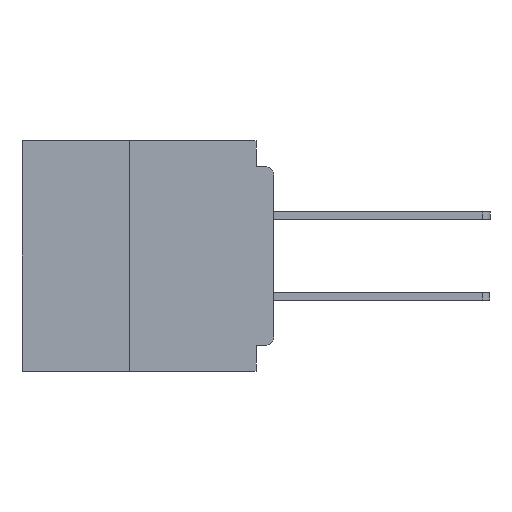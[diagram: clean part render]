
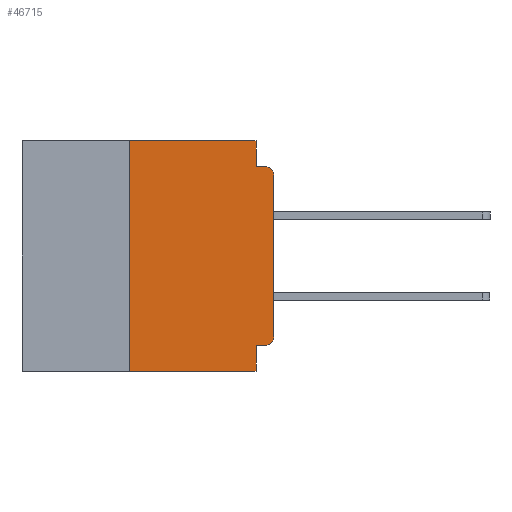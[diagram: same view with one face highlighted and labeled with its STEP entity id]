
A CAD part, left-side view. The second image highlights one B-rep face of the part: STEP entity #46715.
In plain terms, the highlighted planar face has unit normal (-1, 0, 0).
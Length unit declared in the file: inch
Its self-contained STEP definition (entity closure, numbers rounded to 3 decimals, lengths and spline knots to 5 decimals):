
#1260 = ORIENTED_EDGE ( 'NONE', *, *, #4065, .F. ) ;
#1386 = DIRECTION ( 'NONE',  ( 0., 0., -1. ) ) ;
#2509 = CARTESIAN_POINT ( 'NONE',  ( 0., 0.015, -0.355 ) ) ;
#2570 = VERTEX_POINT ( 'NONE', #18987 ) ;
#2714 = LINE ( 'NONE', #21252, #49783 ) ;
#4065 = EDGE_CURVE ( 'NONE', #26588, #33349, #13786, .T. ) ;
#6984 = LINE ( 'NONE', #49546, #52693 ) ;
#7723 = CARTESIAN_POINT ( 'NONE',  ( 0., 0.437, 0. ) ) ;
#8482 = ORIENTED_EDGE ( 'NONE', *, *, #28349, .F. ) ;
#8968 = ORIENTED_EDGE ( 'NONE', *, *, #21781, .T. ) ;
#9814 = LINE ( 'NONE', #50591, #43721 ) ;
#10561 = VERTEX_POINT ( 'NONE', #35014 ) ;
#11578 = VERTEX_POINT ( 'NONE', #30526 ) ;
#11749 = DIRECTION ( 'NONE',  ( 0., 1., 0. ) ) ;
#12349 = EDGE_CURVE ( 'NONE', #39639, #48345, #39547, .T. ) ;
#13540 = LINE ( 'NONE', #41100, #22592 ) ;
#13786 = LINE ( 'NONE', #43522, #46334 ) ;
#15173 = CARTESIAN_POINT ( 'NONE',  ( 0., 0.25, -0.4 ) ) ;
#15641 = DIRECTION ( 'NONE',  ( -1., 0., 0. ) ) ;
#17525 = CARTESIAN_POINT ( 'NONE',  ( 0., 0., -0.045 ) ) ;
#17658 = VERTEX_POINT ( 'NONE', #15173 ) ;
#18987 = CARTESIAN_POINT ( 'NONE',  ( 0., 0.015, -0.045 ) ) ;
#21252 = CARTESIAN_POINT ( 'NONE',  ( 0., 0.25, -0.4 ) ) ;
#21430 = ORIENTED_EDGE ( 'NONE', *, *, #26147, .F. ) ;
#21475 = CARTESIAN_POINT ( 'NONE',  ( 0., 0., 0. ) ) ;
#21781 = EDGE_CURVE ( 'NONE', #17658, #23267, #9814, .T. ) ;
#22251 = EDGE_CURVE ( 'NONE', #10561, #26588, #6984, .T. ) ;
#22592 = VECTOR ( 'NONE', #23510, 39.37008 ) ;
#23130 = EDGE_LOOP ( 'NONE', ( #33157, #50341, #8482, #1260, #29506, #32624, #8968, #35141, #21430, #47176 ) ) ;
#23249 = LINE ( 'NONE', #24923, #57124 ) ;
#23267 = VERTEX_POINT ( 'NONE', #32295 ) ;
#23510 = DIRECTION ( 'NONE',  ( 0., 0., -1. ) ) ;
#24923 = CARTESIAN_POINT ( 'NONE',  ( 0., 0., -0.355 ) ) ;
#25291 = DIRECTION ( 'NONE',  ( 0., 0., 1. ) ) ;
#25569 = PLANE ( 'NONE',  #44986 ) ;
#26147 = EDGE_CURVE ( 'NONE', #39639, #41150, #23249, .T. ) ;
#26588 = VERTEX_POINT ( 'NONE', #54233 ) ;
#27921 = DIRECTION ( 'NONE',  ( -1., 0., 0. ) ) ;
#28349 = EDGE_CURVE ( 'NONE', #33349, #2570, #48219, .T. ) ;
#28579 = EDGE_CURVE ( 'NONE', #41150, #23267, #13540, .T. ) ;
#28597 = CARTESIAN_POINT ( 'NONE',  ( 0., 0.031, -0.045 ) ) ;
#28895 = FACE_OUTER_BOUND ( 'NONE', #23130, .T. ) ;
#29026 = CARTESIAN_POINT ( 'NONE',  ( 0., 0.031, -0.355 ) ) ;
#29506 = ORIENTED_EDGE ( 'NONE', *, *, #22251, .F. ) ;
#30049 = DIRECTION ( 'NONE',  ( 0., 0., -1. ) ) ;
#30526 = CARTESIAN_POINT ( 'NONE',  ( 0., 0., -0.06 ) ) ;
#30920 = DIRECTION ( 'NONE',  ( 0., -1., 0. ) ) ;
#31997 = DIRECTION ( 'NONE',  ( 0., -1., 0. ) ) ;
#32295 = CARTESIAN_POINT ( 'NONE',  ( 0., 0.031, -0.4 ) ) ;
#32624 = ORIENTED_EDGE ( 'NONE', *, *, #51682, .F. ) ;
#33157 = ORIENTED_EDGE ( 'NONE', *, *, #35260, .T. ) ;
#33349 = VERTEX_POINT ( 'NONE', #28597 ) ;
#33749 = VECTOR ( 'NONE', #30920, 39.37008 ) ;
#35014 = CARTESIAN_POINT ( 'NONE',  ( 0., 0.25, 0. ) ) ;
#35064 = EDGE_CURVE ( 'NONE', #11578, #2570, #53491, .T. ) ;
#35141 = ORIENTED_EDGE ( 'NONE', *, *, #28579, .F. ) ;
#35260 = EDGE_CURVE ( 'NONE', #48345, #11578, #42392, .T. ) ;
#37229 = DIRECTION ( 'NONE',  ( 0., -1., 0. ) ) ;
#37273 = AXIS2_PLACEMENT_3D ( 'NONE', #42157, #15641, #46585 ) ;
#39547 = CIRCLE ( 'NONE', #56063, 0.015 ) ;
#39639 = VERTEX_POINT ( 'NONE', #2509 ) ;
#41034 = VECTOR ( 'NONE', #52397, 39.37008 ) ;
#41100 = CARTESIAN_POINT ( 'NONE',  ( 0., 0.031, -0.4 ) ) ;
#41150 = VERTEX_POINT ( 'NONE', #29026 ) ;
#42157 = CARTESIAN_POINT ( 'NONE',  ( 0., 0.015, -0.06 ) ) ;
#42392 = LINE ( 'NONE', #21475, #41034 ) ;
#43522 = CARTESIAN_POINT ( 'NONE',  ( 0., 0.031, 0. ) ) ;
#43708 = DIRECTION ( 'NONE',  ( 0., 0., -1. ) ) ;
#43721 = VECTOR ( 'NONE', #37229, 39.37008 ) ;
#44986 = AXIS2_PLACEMENT_3D ( 'NONE', #7723, #56482, #30049 ) ;
#46334 = VECTOR ( 'NONE', #43708, 39.37008 ) ;
#46585 = DIRECTION ( 'NONE',  ( 0., 0., -1. ) ) ;
#46715 = ADVANCED_FACE ( 'NONE', ( #28895 ), #25569, .F. ) ;
#47176 = ORIENTED_EDGE ( 'NONE', *, *, #12349, .T. ) ;
#48219 = LINE ( 'NONE', #17525, #33749 ) ;
#48345 = VERTEX_POINT ( 'NONE', #50555 ) ;
#49546 = CARTESIAN_POINT ( 'NONE',  ( 0., 0.437, 0. ) ) ;
#49783 = VECTOR ( 'NONE', #25291, 39.37008 ) ;
#50341 = ORIENTED_EDGE ( 'NONE', *, *, #35064, .T. ) ;
#50555 = CARTESIAN_POINT ( 'NONE',  ( 0., 0., -0.34 ) ) ;
#50591 = CARTESIAN_POINT ( 'NONE',  ( 0., 0.437, -0.4 ) ) ;
#51682 = EDGE_CURVE ( 'NONE', #17658, #10561, #2714, .T. ) ;
#52397 = DIRECTION ( 'NONE',  ( 0., 0., 1. ) ) ;
#52693 = VECTOR ( 'NONE', #31997, 39.37008 ) ;
#53491 = CIRCLE ( 'NONE', #37273, 0.015 ) ;
#54233 = CARTESIAN_POINT ( 'NONE',  ( 0., 0.031, 0. ) ) ;
#54354 = CARTESIAN_POINT ( 'NONE',  ( 0., 0.015, -0.34 ) ) ;
#56063 = AXIS2_PLACEMENT_3D ( 'NONE', #54354, #27921, #1386 ) ;
#56482 = DIRECTION ( 'NONE',  ( 1., 0., 0. ) ) ;
#57124 = VECTOR ( 'NONE', #11749, 39.37008 ) ;
